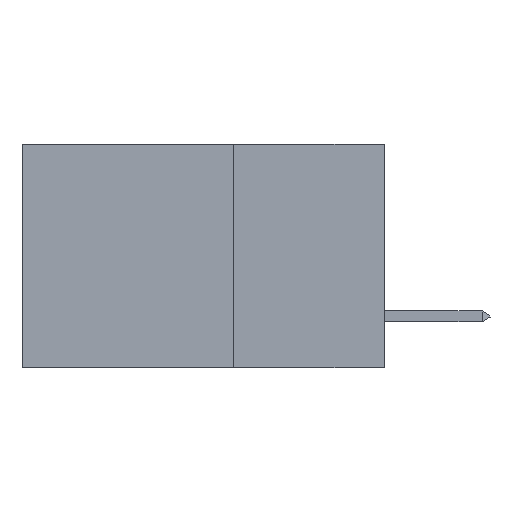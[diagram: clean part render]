
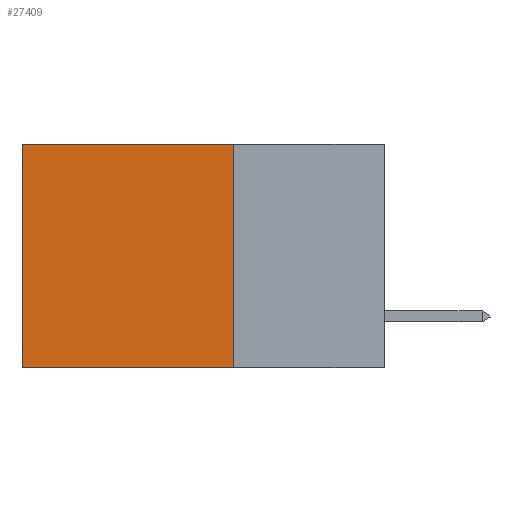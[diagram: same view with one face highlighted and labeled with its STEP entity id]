
A CAD part, left-side view. The second image highlights one B-rep face of the part: STEP entity #27409.
In plain terms, the highlighted planar face has unit normal (-1, 0, 0).
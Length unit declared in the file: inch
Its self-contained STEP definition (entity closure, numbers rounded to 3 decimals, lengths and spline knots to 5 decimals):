
#858 = EDGE_CURVE ( 'NONE', #32296, #27713, #11266, .T. ) ;
#1940 = CARTESIAN_POINT ( 'NONE',  ( 0.2875, 0.25, -0.37 ) ) ;
#4388 = VECTOR ( 'NONE', #27956, 39.37008 ) ;
#5350 = VERTEX_POINT ( 'NONE', #1940 ) ;
#6524 = CARTESIAN_POINT ( 'NONE',  ( 0.2875, 0.25, 0. ) ) ;
#8083 = ORIENTED_EDGE ( 'NONE', *, *, #858, .T. ) ;
#8925 = DIRECTION ( 'NONE',  ( 0., 0., -1. ) ) ;
#9222 = LINE ( 'NONE', #30839, #35775 ) ;
#9510 = CARTESIAN_POINT ( 'NONE',  ( 0.2875, 0.25, 0. ) ) ;
#11266 = LINE ( 'NONE', #17562, #35088 ) ;
#13557 = CARTESIAN_POINT ( 'NONE',  ( 0.2875, 0.6, 0. ) ) ;
#14628 = LINE ( 'NONE', #14824, #4388 ) ;
#14824 = CARTESIAN_POINT ( 'NONE',  ( 0.2875, 0.25, -0.37 ) ) ;
#16830 = EDGE_CURVE ( 'NONE', #18473, #32296, #18075, .T. ) ;
#17223 = DIRECTION ( 'NONE',  ( 0., 0., -1. ) ) ;
#17562 = CARTESIAN_POINT ( 'NONE',  ( 0.2875, 0.6, 0. ) ) ;
#18075 = LINE ( 'NONE', #6524, #36154 ) ;
#18473 = VERTEX_POINT ( 'NONE', #9510 ) ;
#21233 = EDGE_LOOP ( 'NONE', ( #8083, #31163, #24954, #26090 ) ) ;
#22432 = EDGE_CURVE ( 'NONE', #5350, #27713, #14628, .T. ) ;
#23795 = DIRECTION ( 'NONE',  ( 0., 1., 0. ) ) ;
#24954 = ORIENTED_EDGE ( 'NONE', *, *, #27481, .F. ) ;
#25048 = AXIS2_PLACEMENT_3D ( 'NONE', #35183, #32411, #35694 ) ;
#26090 = ORIENTED_EDGE ( 'NONE', *, *, #16830, .T. ) ;
#26505 = PLANE ( 'NONE',  #25048 ) ;
#27409 = ADVANCED_FACE ( 'NONE', ( #30829 ), #26505, .F. ) ;
#27481 = EDGE_CURVE ( 'NONE', #18473, #5350, #9222, .T. ) ;
#27713 = VERTEX_POINT ( 'NONE', #32211 ) ;
#27956 = DIRECTION ( 'NONE',  ( 0., 1., 0. ) ) ;
#30829 = FACE_OUTER_BOUND ( 'NONE', #21233, .T. ) ;
#30839 = CARTESIAN_POINT ( 'NONE',  ( 0.2875, 0.25, 0. ) ) ;
#31163 = ORIENTED_EDGE ( 'NONE', *, *, #22432, .F. ) ;
#32211 = CARTESIAN_POINT ( 'NONE',  ( 0.2875, 0.6, -0.37 ) ) ;
#32296 = VERTEX_POINT ( 'NONE', #13557 ) ;
#32411 = DIRECTION ( 'NONE',  ( 1., 0., 0. ) ) ;
#35088 = VECTOR ( 'NONE', #17223, 39.37008 ) ;
#35183 = CARTESIAN_POINT ( 'NONE',  ( 0.2875, 0.25, 0. ) ) ;
#35694 = DIRECTION ( 'NONE',  ( 0., 0., -1. ) ) ;
#35775 = VECTOR ( 'NONE', #8925, 39.37008 ) ;
#36154 = VECTOR ( 'NONE', #23795, 39.37008 ) ;
